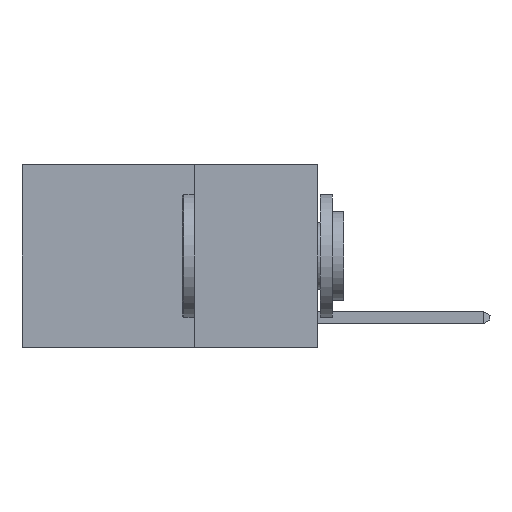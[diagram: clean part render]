
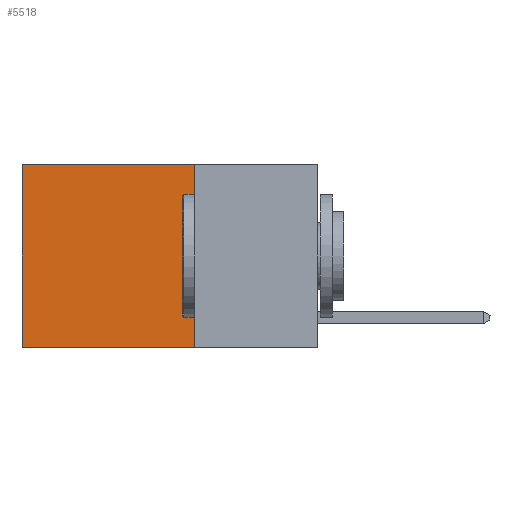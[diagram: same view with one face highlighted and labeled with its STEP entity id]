
A CAD part, left-side view. The second image highlights one B-rep face of the part: STEP entity #5518.
In plain terms, the highlighted planar face has unit normal (-1, 0, 0).
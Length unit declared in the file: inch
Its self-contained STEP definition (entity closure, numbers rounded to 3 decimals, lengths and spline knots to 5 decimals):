
#77 = ORIENTED_EDGE ( 'NONE', *, *, #8380, .F. ) ;
#238 = CARTESIAN_POINT ( 'NONE',  ( 0.2625, 0.25, -0.37 ) ) ;
#710 = DIRECTION ( 'NONE',  ( 0., 0., -1. ) ) ;
#879 = DIRECTION ( 'NONE',  ( 0., 1., 0. ) ) ;
#1381 = ORIENTED_EDGE ( 'NONE', *, *, #5174, .T. ) ;
#1385 = LINE ( 'NONE', #7761, #8062 ) ;
#1894 = DIRECTION ( 'NONE',  ( 0., 1., 0. ) ) ;
#1992 = CARTESIAN_POINT ( 'NONE',  ( 0.2625, 0.25, 0. ) ) ;
#1998 = CARTESIAN_POINT ( 'NONE',  ( 0.2625, 0.25, 0. ) ) ;
#2101 = EDGE_CURVE ( 'NONE', #5151, #9274, #6461, .T. ) ;
#2103 = VECTOR ( 'NONE', #879, 39.37008 ) ;
#2393 = DIRECTION ( 'NONE',  ( 0., 0., -1. ) ) ;
#3123 = LINE ( 'NONE', #7125, #7376 ) ;
#3220 = DIRECTION ( 'NONE',  ( 0., 0., -1. ) ) ;
#3799 = CARTESIAN_POINT ( 'NONE',  ( 0.2625, 0.6, -0.37 ) ) ;
#4135 = CARTESIAN_POINT ( 'NONE',  ( 0.2625, 0.25, -0.37 ) ) ;
#4252 = VERTEX_POINT ( 'NONE', #5537 ) ;
#4897 = EDGE_CURVE ( 'NONE', #4252, #9274, #1385, .T. ) ;
#5151 = VERTEX_POINT ( 'NONE', #238 ) ;
#5174 = EDGE_CURVE ( 'NONE', #8536, #4252, #8949, .T. ) ;
#5455 = PLANE ( 'NONE',  #5847 ) ;
#5518 = ADVANCED_FACE ( 'NONE', ( #9401 ), #5455, .F. ) ;
#5537 = CARTESIAN_POINT ( 'NONE',  ( 0.2625, 0.6, 0. ) ) ;
#5750 = ORIENTED_EDGE ( 'NONE', *, *, #4897, .T. ) ;
#5847 = AXIS2_PLACEMENT_3D ( 'NONE', #6283, #9444, #2393 ) ;
#6016 = EDGE_LOOP ( 'NONE', ( #5750, #6753, #77, #1381 ) ) ;
#6283 = CARTESIAN_POINT ( 'NONE',  ( 0.2625, 0.25, 0. ) ) ;
#6461 = LINE ( 'NONE', #4135, #2103 ) ;
#6753 = ORIENTED_EDGE ( 'NONE', *, *, #2101, .F. ) ;
#7125 = CARTESIAN_POINT ( 'NONE',  ( 0.2625, 0.25, 0. ) ) ;
#7376 = VECTOR ( 'NONE', #3220, 39.37008 ) ;
#7761 = CARTESIAN_POINT ( 'NONE',  ( 0.2625, 0.6, 0. ) ) ;
#8062 = VECTOR ( 'NONE', #710, 39.37008 ) ;
#8380 = EDGE_CURVE ( 'NONE', #8536, #5151, #3123, .T. ) ;
#8536 = VERTEX_POINT ( 'NONE', #1992 ) ;
#8949 = LINE ( 'NONE', #1998, #9482 ) ;
#9274 = VERTEX_POINT ( 'NONE', #3799 ) ;
#9401 = FACE_OUTER_BOUND ( 'NONE', #6016, .T. ) ;
#9444 = DIRECTION ( 'NONE',  ( 1., 0., 0. ) ) ;
#9482 = VECTOR ( 'NONE', #1894, 39.37008 ) ;
